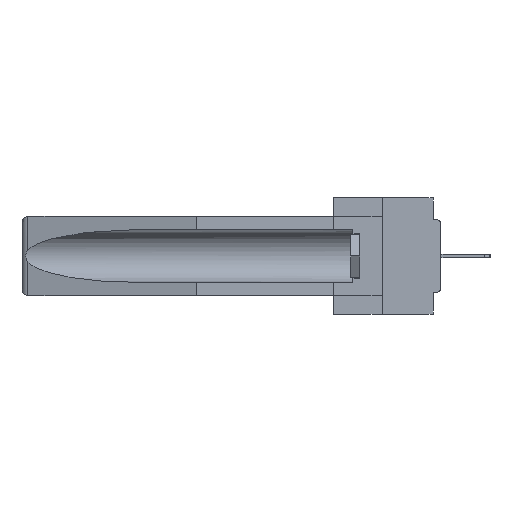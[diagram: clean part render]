
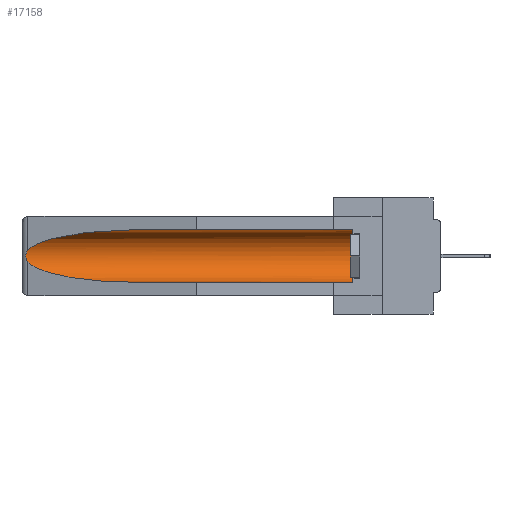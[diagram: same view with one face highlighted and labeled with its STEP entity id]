
A CAD part, left-side view. The second image highlights one B-rep face of the part: STEP entity #17158.
In plain terms, the highlighted cylindrical face has radius 2.857 mm (diameter 5.715 mm), a partial arc.
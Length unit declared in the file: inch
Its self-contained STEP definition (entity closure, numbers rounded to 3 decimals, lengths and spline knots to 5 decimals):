
#244 = CARTESIAN_POINT ( 'NONE',  ( 0.26537, 1.52718, -0.14972 ) ) ;
#503 = ORIENTED_EDGE ( 'NONE', *, *, #1383, .F. ) ;
#757 = DIRECTION ( 'NONE',  ( 0., 1., 0. ) ) ;
#1383 = EDGE_CURVE ( 'NONE', #21894, #11918, #9332, .T. ) ;
#2221 = CARTESIAN_POINT ( 'NONE',  ( 0.2673, 1.53269, -0.17917 ) ) ;
#2600 = ORIENTED_EDGE ( 'NONE', *, *, #25418, .T. ) ;
#4111 = ORIENTED_EDGE ( 'NONE', *, *, #11633, .T. ) ;
#4311 = CARTESIAN_POINT ( 'NONE',  ( 0.25451, 1.48313, -0.24835 ) ) ;
#5282 = CARTESIAN_POINT ( 'NONE',  ( 0.26597, 1.5296, -0.19026 ) ) ;
#6445 = CARTESIAN_POINT ( 'NONE',  ( 0.155, 1.07973, -0.284 ) ) ;
#6774 = CARTESIAN_POINT ( 'NONE',  ( 0.26537, 1.52718, -0.14972 ) ) ;
#7353 = CARTESIAN_POINT ( 'NONE',  ( 0.21114, 1.30732, -0.284 ) ) ;
#8255 = EDGE_LOOP ( 'NONE', ( #31120, #4111, #2600, #503, #17479, #14642 ) ) ;
#8281 = EDGE_CURVE ( 'NONE', #16895, #25341, #13150, .T. ) ;
#8496 = VERTEX_POINT ( 'NONE', #244 ) ;
#8538 = CARTESIAN_POINT ( 'NONE',  ( 0.155, -0.30754, -0.284 ) ) ;
#9332 = LINE ( 'NONE', #8538, #17467 ) ;
#9960 =( BOUNDED_CURVE ( )  B_SPLINE_CURVE ( 3, ( #21949, #33806, #24921, #6774 ),
 .UNSPECIFIED., .F., .T. ) 
 B_SPLINE_CURVE_WITH_KNOTS ( ( 4, 4 ),
 ( 4.71239, 6.08839 ),
 .UNSPECIFIED. ) 
 CURVE ( )  GEOMETRIC_REPRESENTATION_ITEM ( )  RATIONAL_B_SPLINE_CURVE ( ( 1., 0.848, 0.848, 1. ) ) 
 REPRESENTATION_ITEM ( '' )  );
#11365 = CARTESIAN_POINT ( 'NONE',  ( 0.155, -0.30754, -0.059 ) ) ;
#11633 = EDGE_CURVE ( 'NONE', #8496, #31851, #38402, .T. ) ;
#11918 = VERTEX_POINT ( 'NONE', #6445 ) ;
#13150 = LINE ( 'NONE', #11365, #28162 ) ;
#14642 = ORIENTED_EDGE ( 'NONE', *, *, #8281, .T. ) ;
#16895 = VERTEX_POINT ( 'NONE', #38831 ) ;
#17129 = EDGE_CURVE ( 'NONE', #25341, #8496, #9960, .T. ) ;
#17158 = ADVANCED_FACE ( 'NONE', ( #23846 ), #22924, .F. ) ;
#17446 = CARTESIAN_POINT ( 'NONE',  ( 0.2673, 1.5327, -0.16383 ) ) ;
#17467 = VECTOR ( 'NONE', #35663, 39.37008 ) ;
#17479 = ORIENTED_EDGE ( 'NONE', *, *, #21800, .T. ) ;
#17517 =( BOUNDED_CURVE ( )  B_SPLINE_CURVE ( 3, ( #31220, #4311, #7353, #28473 ),
 .UNSPECIFIED., .F., .F. ) 
 B_SPLINE_CURVE_WITH_KNOTS ( ( 4, 4 ),
 ( 0.1948, 1.5708 ),
 .UNSPECIFIED. ) 
 CURVE ( )  GEOMETRIC_REPRESENTATION_ITEM ( )  RATIONAL_B_SPLINE_CURVE ( ( 1., 0.848, 0.848, 1. ) ) 
 REPRESENTATION_ITEM ( '' )  );
#17817 = CARTESIAN_POINT ( 'NONE',  ( 0.155, 0.126, -0.1715 ) ) ;
#18465 = CIRCLE ( 'NONE', #37348, 0.1125 ) ;
#19063 = CARTESIAN_POINT ( 'NONE',  ( 0.155, -0.30754, -0.1715 ) ) ;
#20477 = CARTESIAN_POINT ( 'NONE',  ( 0.2675, 1.53308, -0.17534 ) ) ;
#20847 = DIRECTION ( 'NONE',  ( 0., 0., 1. ) ) ;
#21800 = EDGE_CURVE ( 'NONE', #21894, #16895, #18465, .T. ) ;
#21894 = VERTEX_POINT ( 'NONE', #29922 ) ;
#21949 = CARTESIAN_POINT ( 'NONE',  ( 0.155, 1.07973, -0.059 ) ) ;
#22081 = DIRECTION ( 'NONE',  ( 0., 0., 1. ) ) ;
#22924 = CYLINDRICAL_SURFACE ( 'NONE', #37235, 0.1125 ) ;
#23492 = CARTESIAN_POINT ( 'NONE',  ( 0.26655, 1.53094, -0.18657 ) ) ;
#23846 = FACE_OUTER_BOUND ( 'NONE', #8255, .T. ) ;
#24921 = CARTESIAN_POINT ( 'NONE',  ( 0.25451, 1.48313, -0.09465 ) ) ;
#25341 = VERTEX_POINT ( 'NONE', #34004 ) ;
#25418 = EDGE_CURVE ( 'NONE', #31851, #11918, #17517, .T. ) ;
#26457 = CARTESIAN_POINT ( 'NONE',  ( 0.26537, 1.52718, -0.19328 ) ) ;
#27165 = CARTESIAN_POINT ( 'NONE',  ( 0.26537, 1.52718, -0.19328 ) ) ;
#28162 = VECTOR ( 'NONE', #32404, 39.37008 ) ;
#28473 = CARTESIAN_POINT ( 'NONE',  ( 0.155, 1.07973, -0.284 ) ) ;
#29922 = CARTESIAN_POINT ( 'NONE',  ( 0.155, 0.126, -0.284 ) ) ;
#31120 = ORIENTED_EDGE ( 'NONE', *, *, #17129, .T. ) ;
#31220 = CARTESIAN_POINT ( 'NONE',  ( 0.26537, 1.52718, -0.19328 ) ) ;
#31851 = VERTEX_POINT ( 'NONE', #27165 ) ;
#32332 = CARTESIAN_POINT ( 'NONE',  ( 0.26537, 1.52718, -0.14972 ) ) ;
#32404 = DIRECTION ( 'NONE',  ( 0., 1., 0. ) ) ;
#33806 = CARTESIAN_POINT ( 'NONE',  ( 0.21114, 1.30732, -0.059 ) ) ;
#34004 = CARTESIAN_POINT ( 'NONE',  ( 0.155, 1.07973, -0.059 ) ) ;
#35354 = CARTESIAN_POINT ( 'NONE',  ( 0.26654, 1.53092, -0.15636 ) ) ;
#35663 = DIRECTION ( 'NONE',  ( 0., 1., 0. ) ) ;
#37235 = AXIS2_PLACEMENT_3D ( 'NONE', #19063, #757, #22081 ) ;
#37348 = AXIS2_PLACEMENT_3D ( 'NONE', #17817, #38757, #20847 ) ;
#38257 = CARTESIAN_POINT ( 'NONE',  ( 0.26597, 1.52961, -0.15275 ) ) ;
#38392 = CARTESIAN_POINT ( 'NONE',  ( 0.2675, 1.53308, -0.16763 ) ) ;
#38402 = B_SPLINE_CURVE_WITH_KNOTS ( 'NONE', 3,
 ( #32332, #38257, #35354, #17446, #38392, #20477, #2221, #23492, #5282, #26457 ),
 .UNSPECIFIED., .F., .F.,
 ( 4, 2, 2, 2, 4 ),
 ( 0., 0.00029, 0.00058, 0.00087, 0.00117 ),
 .UNSPECIFIED. ) ;
#38757 = DIRECTION ( 'NONE',  ( 0., -1., 0. ) ) ;
#38831 = CARTESIAN_POINT ( 'NONE',  ( 0.155, 0.126, -0.059 ) ) ;
